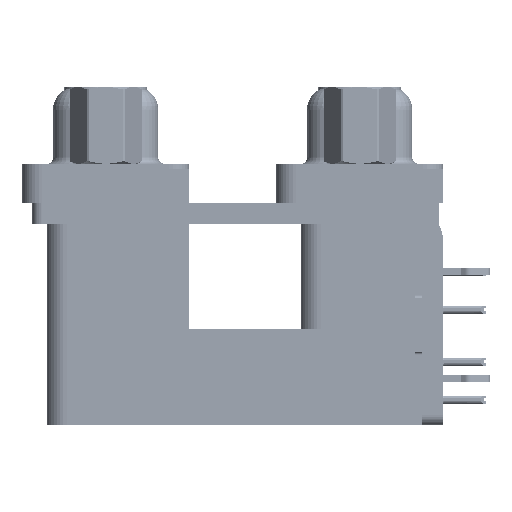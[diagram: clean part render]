
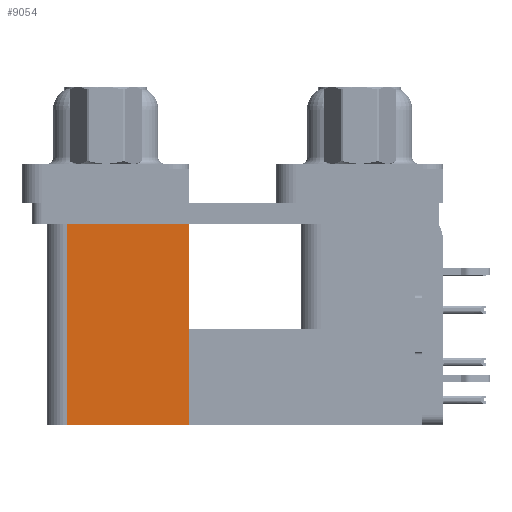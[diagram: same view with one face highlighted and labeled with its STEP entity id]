
A CAD part, left-side view. The second image highlights one B-rep face of the part: STEP entity #9054.
In plain terms, the highlighted planar face has unit normal (-1, 0, 0).
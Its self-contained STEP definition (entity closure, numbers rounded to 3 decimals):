
#790 = PLANE ( 'NONE',  #25775 ) ;
#3690 = VECTOR ( 'NONE', #28005, 1000. ) ;
#9050 = ORIENTED_EDGE ( 'NONE', *, *, #26579, .F. ) ;
#9054 = ADVANCED_FACE ( 'NONE', ( #38191 ), #790, .F. ) ;
#9428 = LINE ( 'NONE', #30357, #63029 ) ;
#10736 = ORIENTED_EDGE ( 'NONE', *, *, #38367, .F. ) ;
#11738 = CARTESIAN_POINT ( 'NONE',  ( 3.7, 12.775, -19.2 ) ) ;
#14625 = VECTOR ( 'NONE', #15768, 1000. ) ;
#15768 = DIRECTION ( 'NONE',  ( 0., 0., 1. ) ) ;
#19253 = CARTESIAN_POINT ( 'NONE',  ( 3.7, 12.775, -19.2 ) ) ;
#20145 = ORIENTED_EDGE ( 'NONE', *, *, #41546, .T. ) ;
#24162 = CARTESIAN_POINT ( 'NONE',  ( 3.7, 12.775, -2.5 ) ) ;
#25775 = AXIS2_PLACEMENT_3D ( 'NONE', #11738, #42697, #38528 ) ;
#26579 = EDGE_CURVE ( 'NONE', #62625, #63309, #54027, .T. ) ;
#27650 = CARTESIAN_POINT ( 'NONE',  ( 3.7, 21.975, -2.5 ) ) ;
#28005 = DIRECTION ( 'NONE',  ( 0., 0., 1. ) ) ;
#28933 = CARTESIAN_POINT ( 'NONE',  ( 3.7, 12.775, -19.2 ) ) ;
#30357 = CARTESIAN_POINT ( 'NONE',  ( 3.7, 12.775, -2.5 ) ) ;
#32907 = VERTEX_POINT ( 'NONE', #24162 ) ;
#37783 = VERTEX_POINT ( 'NONE', #27650 ) ;
#38083 = CARTESIAN_POINT ( 'NONE',  ( 3.7, 21.975, -19.2 ) ) ;
#38191 = FACE_OUTER_BOUND ( 'NONE', #67503, .T. ) ;
#38367 = EDGE_CURVE ( 'NONE', #63309, #37783, #62856, .T. ) ;
#38528 = DIRECTION ( 'NONE',  ( 0., 1., 0. ) ) ;
#39698 = DIRECTION ( 'NONE',  ( 0., 1., 0. ) ) ;
#40116 = EDGE_CURVE ( 'NONE', #62625, #32907, #48671, .T. ) ;
#41546 = EDGE_CURVE ( 'NONE', #32907, #37783, #9428, .T. ) ;
#42528 = VECTOR ( 'NONE', #55385, 1000. ) ;
#42697 = DIRECTION ( 'NONE',  ( 1., 0., 0. ) ) ;
#48671 = LINE ( 'NONE', #53507, #3690 ) ;
#53507 = CARTESIAN_POINT ( 'NONE',  ( 3.7, 12.775, -19.2 ) ) ;
#54027 = LINE ( 'NONE', #19253, #42528 ) ;
#55385 = DIRECTION ( 'NONE',  ( 0., 1., 0. ) ) ;
#57031 = CARTESIAN_POINT ( 'NONE',  ( 3.7, 21.975, -19.2 ) ) ;
#62625 = VERTEX_POINT ( 'NONE', #28933 ) ;
#62856 = LINE ( 'NONE', #57031, #14625 ) ;
#63029 = VECTOR ( 'NONE', #39698, 1000. ) ;
#63309 = VERTEX_POINT ( 'NONE', #38083 ) ;
#65903 = ORIENTED_EDGE ( 'NONE', *, *, #40116, .T. ) ;
#67503 = EDGE_LOOP ( 'NONE', ( #20145, #10736, #9050, #65903 ) ) ;
